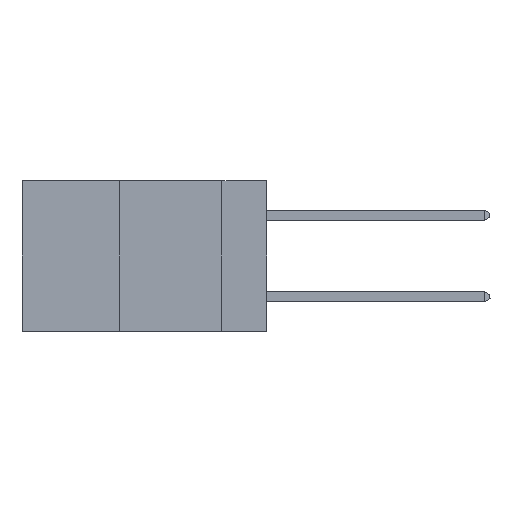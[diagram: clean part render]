
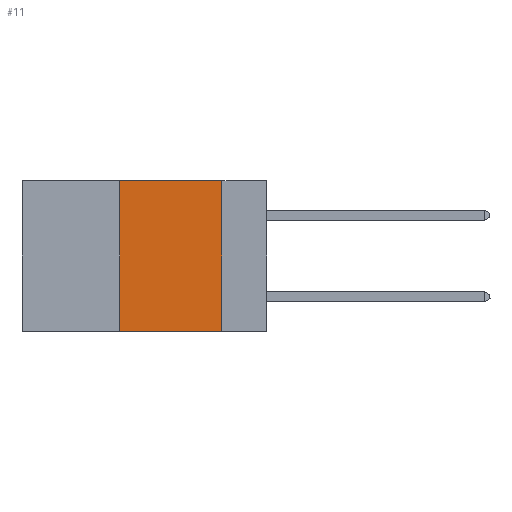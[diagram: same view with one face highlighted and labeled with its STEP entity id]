
A CAD part, left-side view. The second image highlights one B-rep face of the part: STEP entity #11.
In plain terms, the highlighted planar face has unit normal (-1, 0, 0).
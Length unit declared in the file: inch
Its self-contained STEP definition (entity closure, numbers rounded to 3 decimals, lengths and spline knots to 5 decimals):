
#11 = ADVANCED_FACE ( 'NONE', ( #6790 ), #10514, .F. ) ;
#539 = EDGE_CURVE ( 'NONE', #12519, #12758, #11323, .T. ) ;
#734 = DIRECTION ( 'NONE',  ( 0., 0., -1. ) ) ;
#2101 = ORIENTED_EDGE ( 'NONE', *, *, #4153, .F. ) ;
#2390 = ORIENTED_EDGE ( 'NONE', *, *, #12441, .F. ) ;
#3077 = VERTEX_POINT ( 'NONE', #6449 ) ;
#4153 = EDGE_CURVE ( 'NONE', #12519, #9762, #6171, .T. ) ;
#4293 = EDGE_LOOP ( 'NONE', ( #4792, #2390, #2101, #7600 ) ) ;
#4792 = ORIENTED_EDGE ( 'NONE', *, *, #6521, .F. ) ;
#6171 = LINE ( 'NONE', #11047, #11067 ) ;
#6235 = VECTOR ( 'NONE', #7867, 39.37008 ) ;
#6449 = CARTESIAN_POINT ( 'NONE',  ( 0., 0.11, 0. ) ) ;
#6521 = EDGE_CURVE ( 'NONE', #3077, #12758, #12061, .T. ) ;
#6790 = FACE_OUTER_BOUND ( 'NONE', #4293, .T. ) ;
#7096 = CARTESIAN_POINT ( 'NONE',  ( 0., 0.36, 0. ) ) ;
#7600 = ORIENTED_EDGE ( 'NONE', *, *, #539, .T. ) ;
#7867 = DIRECTION ( 'NONE',  ( 0., -1., 0. ) ) ;
#8808 = VECTOR ( 'NONE', #11117, 39.37008 ) ;
#9598 = CARTESIAN_POINT ( 'NONE',  ( 0., 0.6, 0. ) ) ;
#9762 = VERTEX_POINT ( 'NONE', #7096 ) ;
#9811 = CARTESIAN_POINT ( 'NONE',  ( 0., 0.6, 0. ) ) ;
#9896 = CARTESIAN_POINT ( 'NONE',  ( 0., 0.36, -0.37 ) ) ;
#10118 = VECTOR ( 'NONE', #12103, 39.37008 ) ;
#10234 = AXIS2_PLACEMENT_3D ( 'NONE', #9598, #11423, #734 ) ;
#10514 = PLANE ( 'NONE',  #10234 ) ;
#10798 = DIRECTION ( 'NONE',  ( 0., 0., 1. ) ) ;
#10882 = CARTESIAN_POINT ( 'NONE',  ( 0., 0.6, -0.37 ) ) ;
#11047 = CARTESIAN_POINT ( 'NONE',  ( 0., 0.36, 0. ) ) ;
#11067 = VECTOR ( 'NONE', #10798, 39.37008 ) ;
#11117 = DIRECTION ( 'NONE',  ( 0., -1., 0. ) ) ;
#11323 = LINE ( 'NONE', #10882, #8808 ) ;
#11414 = LINE ( 'NONE', #9811, #6235 ) ;
#11423 = DIRECTION ( 'NONE',  ( 1., 0., 0. ) ) ;
#12061 = LINE ( 'NONE', #12197, #10118 ) ;
#12103 = DIRECTION ( 'NONE',  ( 0., 0., -1. ) ) ;
#12197 = CARTESIAN_POINT ( 'NONE',  ( 0., 0.11, 0. ) ) ;
#12316 = CARTESIAN_POINT ( 'NONE',  ( 0., 0.11, -0.37 ) ) ;
#12441 = EDGE_CURVE ( 'NONE', #9762, #3077, #11414, .T. ) ;
#12519 = VERTEX_POINT ( 'NONE', #9896 ) ;
#12758 = VERTEX_POINT ( 'NONE', #12316 ) ;
